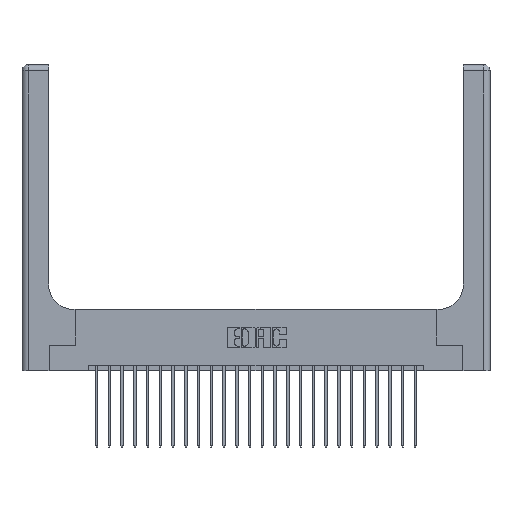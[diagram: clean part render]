
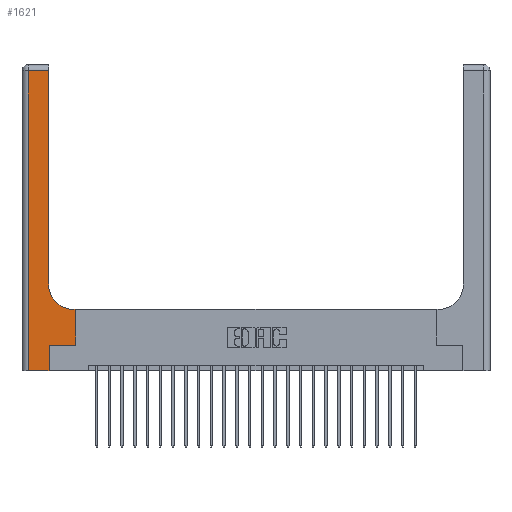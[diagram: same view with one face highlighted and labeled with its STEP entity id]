
A CAD part, top view. The second image highlights one B-rep face of the part: STEP entity #1621.
In plain terms, the highlighted planar face has unit normal (0, 0, 1).
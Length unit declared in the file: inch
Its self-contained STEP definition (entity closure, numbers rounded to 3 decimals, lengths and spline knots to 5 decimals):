
#483 = ORIENTED_EDGE ( 'NONE', *, *, #17783, .T. ) ;
#485 = EDGE_CURVE ( 'NONE', #632, #23626, #5480, .T. ) ;
#632 = VERTEX_POINT ( 'NONE', #18911 ) ;
#861 = ORIENTED_EDGE ( 'NONE', *, *, #13863, .T. ) ;
#952 = DIRECTION ( 'NONE',  ( 0., 0., -1. ) ) ;
#1621 = ADVANCED_FACE ( 'NONE', ( #14437 ), #20033, .F. ) ;
#2299 = LINE ( 'NONE', #19484, #15756 ) ;
#2503 = LINE ( 'NONE', #8299, #20559 ) ;
#2887 = CARTESIAN_POINT ( 'NONE',  ( 0.06, 3., 0.37 ) ) ;
#3211 = CARTESIAN_POINT ( 'NONE',  ( 0.26, 0.85, 0.37 ) ) ;
#3231 = CARTESIAN_POINT ( 'NONE',  ( 0.51, 0.6, 0.37 ) ) ;
#3462 = ORIENTED_EDGE ( 'NONE', *, *, #17119, .T. ) ;
#4507 = DIRECTION ( 'NONE',  ( 1., 0., 0. ) ) ;
#4583 = ORIENTED_EDGE ( 'NONE', *, *, #11888, .T. ) ;
#4606 = EDGE_CURVE ( 'NONE', #11371, #13861, #7112, .T. ) ;
#4772 = CARTESIAN_POINT ( 'NONE',  ( 0.06, 0., 0.37 ) ) ;
#4785 = DIRECTION ( 'NONE',  ( 0., -1., 0. ) ) ;
#4817 = CARTESIAN_POINT ( 'NONE',  ( 0.528, 0.25, 0.37 ) ) ;
#5234 = CARTESIAN_POINT ( 'NONE',  ( 0., 2.94, 0.37 ) ) ;
#5480 = LINE ( 'NONE', #24517, #18375 ) ;
#5515 = CARTESIAN_POINT ( 'NONE',  ( 0.51, 0.85, 0.37 ) ) ;
#5971 = VERTEX_POINT ( 'NONE', #10948 ) ;
#6379 = AXIS2_PLACEMENT_3D ( 'NONE', #14309, #952, #18311 ) ;
#7112 = LINE ( 'NONE', #5234, #14160 ) ;
#8103 = AXIS2_PLACEMENT_3D ( 'NONE', #5515, #11684, #19074 ) ;
#8299 = CARTESIAN_POINT ( 'NONE',  ( 0.265, 0., 0.37 ) ) ;
#8536 = LINE ( 'NONE', #18220, #24332 ) ;
#8954 = VERTEX_POINT ( 'NONE', #3211 ) ;
#10948 = CARTESIAN_POINT ( 'NONE',  ( 0.265, 0., 0.37 ) ) ;
#11270 = DIRECTION ( 'NONE',  ( 0., 1., 0. ) ) ;
#11371 = VERTEX_POINT ( 'NONE', #17844 ) ;
#11397 = VERTEX_POINT ( 'NONE', #4772 ) ;
#11684 = DIRECTION ( 'NONE',  ( 0., 0., -1. ) ) ;
#11888 = EDGE_CURVE ( 'NONE', #13249, #632, #2299, .T. ) ;
#12076 = LINE ( 'NONE', #2887, #22846 ) ;
#12348 = EDGE_CURVE ( 'NONE', #5971, #13177, #2503, .T. ) ;
#12907 = ORIENTED_EDGE ( 'NONE', *, *, #485, .T. ) ;
#13004 = ORIENTED_EDGE ( 'NONE', *, *, #12348, .T. ) ;
#13039 = DIRECTION ( 'NONE',  ( -1., 0., 0. ) ) ;
#13177 = VERTEX_POINT ( 'NONE', #22099 ) ;
#13249 = VERTEX_POINT ( 'NONE', #4817 ) ;
#13563 = VECTOR ( 'NONE', #11270, 39.37008 ) ;
#13861 = VERTEX_POINT ( 'NONE', #21175 ) ;
#13863 = EDGE_CURVE ( 'NONE', #23626, #8954, #20891, .T. ) ;
#14108 = ORIENTED_EDGE ( 'NONE', *, *, #18495, .T. ) ;
#14160 = VECTOR ( 'NONE', #13039, 39.37008 ) ;
#14309 = CARTESIAN_POINT ( 'NONE',  ( 0., 3., 0.37 ) ) ;
#14437 = FACE_OUTER_BOUND ( 'NONE', #17236, .T. ) ;
#14557 = DIRECTION ( 'NONE',  ( 0., 1., 0. ) ) ;
#14904 = ORIENTED_EDGE ( 'NONE', *, *, #4606, .T. ) ;
#15756 = VECTOR ( 'NONE', #17635, 39.37008 ) ;
#16240 = ORIENTED_EDGE ( 'NONE', *, *, #21351, .T. ) ;
#17119 = EDGE_CURVE ( 'NONE', #13177, #13249, #8536, .T. ) ;
#17236 = EDGE_LOOP ( 'NONE', ( #16240, #14904, #14108, #483, #13004, #3462, #4583, #12907, #861 ) ) ;
#17635 = DIRECTION ( 'NONE',  ( 0., 1., 0. ) ) ;
#17783 = EDGE_CURVE ( 'NONE', #11397, #5971, #20496, .T. ) ;
#17844 = CARTESIAN_POINT ( 'NONE',  ( 0.26, 2.94, 0.37 ) ) ;
#18220 = CARTESIAN_POINT ( 'NONE',  ( 0.265, 0.25, 0.37 ) ) ;
#18311 = DIRECTION ( 'NONE',  ( -1., 0., 0. ) ) ;
#18375 = VECTOR ( 'NONE', #24033, 39.37008 ) ;
#18456 = VECTOR ( 'NONE', #24754, 39.37008 ) ;
#18495 = EDGE_CURVE ( 'NONE', #13861, #11397, #12076, .T. ) ;
#18911 = CARTESIAN_POINT ( 'NONE',  ( 0.528, 0.6, 0.37 ) ) ;
#19074 = DIRECTION ( 'NONE',  ( 1., 0., 0. ) ) ;
#19378 = CARTESIAN_POINT ( 'NONE',  ( 0.26, 3., 0.37 ) ) ;
#19484 = CARTESIAN_POINT ( 'NONE',  ( 0.528, 0.25, 0.37 ) ) ;
#20033 = PLANE ( 'NONE',  #6379 ) ;
#20496 = LINE ( 'NONE', #20616, #18456 ) ;
#20559 = VECTOR ( 'NONE', #14557, 39.37008 ) ;
#20616 = CARTESIAN_POINT ( 'NONE',  ( 0., 0., 0.37 ) ) ;
#20891 = CIRCLE ( 'NONE', #8103, 0.25 ) ;
#21175 = CARTESIAN_POINT ( 'NONE',  ( 0.06, 2.94, 0.37 ) ) ;
#21351 = EDGE_CURVE ( 'NONE', #8954, #11371, #22771, .T. ) ;
#22099 = CARTESIAN_POINT ( 'NONE',  ( 0.265, 0.25, 0.37 ) ) ;
#22771 = LINE ( 'NONE', #19378, #13563 ) ;
#22846 = VECTOR ( 'NONE', #4785, 39.37008 ) ;
#23626 = VERTEX_POINT ( 'NONE', #3231 ) ;
#24033 = DIRECTION ( 'NONE',  ( -1., 0., 0. ) ) ;
#24332 = VECTOR ( 'NONE', #4507, 39.37008 ) ;
#24517 = CARTESIAN_POINT ( 'NONE',  ( 0.26, 0.6, 0.37 ) ) ;
#24754 = DIRECTION ( 'NONE',  ( 1., 0., 0. ) ) ;
